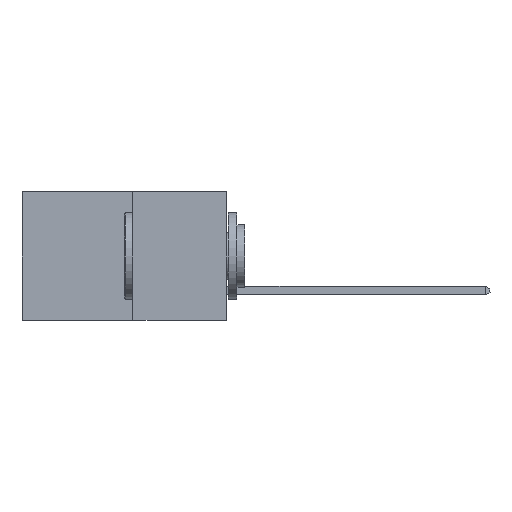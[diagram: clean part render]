
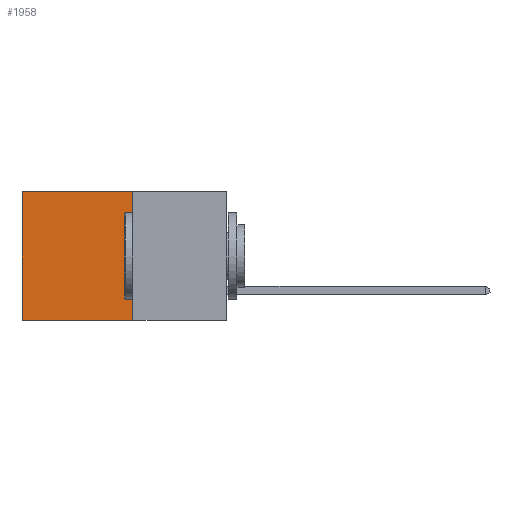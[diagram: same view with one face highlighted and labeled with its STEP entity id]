
A CAD part, left-side view. The second image highlights one B-rep face of the part: STEP entity #1958.
In plain terms, the highlighted planar face has unit normal (-1, 0, 0).
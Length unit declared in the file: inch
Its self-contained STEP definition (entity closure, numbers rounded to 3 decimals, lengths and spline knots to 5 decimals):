
#180 = CARTESIAN_POINT ( 'NONE',  ( 0.277, 0.27, 0. ) ) ;
#1074 = ORIENTED_EDGE ( 'NONE', *, *, #7276, .T. ) ;
#1105 = CARTESIAN_POINT ( 'NONE',  ( 0.277, 0.27, 0. ) ) ;
#1128 = ORIENTED_EDGE ( 'NONE', *, *, #6887, .F. ) ;
#1143 = EDGE_LOOP ( 'NONE', ( #1074, #1128, #1174, #1181 ) ) ;
#1174 = ORIENTED_EDGE ( 'NONE', *, *, #4602, .F. ) ;
#1181 = ORIENTED_EDGE ( 'NONE', *, *, #11178, .T. ) ;
#1652 = AXIS2_PLACEMENT_3D ( 'NONE', #2217, #3908, #5373 ) ;
#1724 = DIRECTION ( 'NONE',  ( 0., 1., 0. ) ) ;
#1958 = ADVANCED_FACE ( 'NONE', ( #10789 ), #5033, .F. ) ;
#1964 = CARTESIAN_POINT ( 'NONE',  ( 0.277, 0.59, 0. ) ) ;
#2217 = CARTESIAN_POINT ( 'NONE',  ( 0.277, 0.27, -0.37 ) ) ;
#2432 = VERTEX_POINT ( 'NONE', #4342 ) ;
#2550 = VECTOR ( 'NONE', #1724, 39.37008 ) ;
#2696 = VECTOR ( 'NONE', #8814, 39.37008 ) ;
#3224 = VECTOR ( 'NONE', #9479, 39.37008 ) ;
#3908 = DIRECTION ( 'NONE',  ( 1., 0., 0. ) ) ;
#4113 = VERTEX_POINT ( 'NONE', #1964 ) ;
#4342 = CARTESIAN_POINT ( 'NONE',  ( 0.277, 0.27, -0.37 ) ) ;
#4602 = EDGE_CURVE ( 'NONE', #6814, #2432, #5836, .T. ) ;
#5033 = PLANE ( 'NONE',  #1652 ) ;
#5373 = DIRECTION ( 'NONE',  ( 0., 0., -1. ) ) ;
#5613 = LINE ( 'NONE', #6203, #2696 ) ;
#5743 = VECTOR ( 'NONE', #5986, 39.37008 ) ;
#5836 = LINE ( 'NONE', #9765, #3224 ) ;
#5986 = DIRECTION ( 'NONE',  ( 0., 1., 0. ) ) ;
#6203 = CARTESIAN_POINT ( 'NONE',  ( 0.277, 0.59, -0.37 ) ) ;
#6814 = VERTEX_POINT ( 'NONE', #180 ) ;
#6887 = EDGE_CURVE ( 'NONE', #2432, #9761, #9595, .T. ) ;
#7270 = CARTESIAN_POINT ( 'NONE',  ( 0.277, 0.59, -0.37 ) ) ;
#7276 = EDGE_CURVE ( 'NONE', #4113, #9761, #5613, .T. ) ;
#7434 = CARTESIAN_POINT ( 'NONE',  ( 0.277, 0.27, -0.37 ) ) ;
#8098 = LINE ( 'NONE', #1105, #5743 ) ;
#8814 = DIRECTION ( 'NONE',  ( 0., 0., -1. ) ) ;
#9479 = DIRECTION ( 'NONE',  ( 0., 0., -1. ) ) ;
#9595 = LINE ( 'NONE', #7434, #2550 ) ;
#9761 = VERTEX_POINT ( 'NONE', #7270 ) ;
#9765 = CARTESIAN_POINT ( 'NONE',  ( 0.277, 0.27, -0.37 ) ) ;
#10789 = FACE_OUTER_BOUND ( 'NONE', #1143, .T. ) ;
#11178 = EDGE_CURVE ( 'NONE', #6814, #4113, #8098, .T. ) ;
